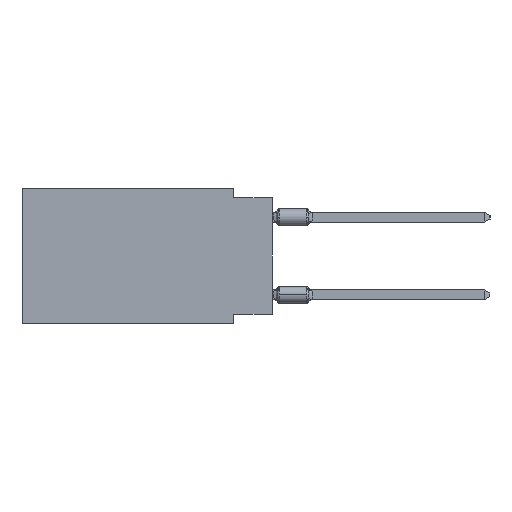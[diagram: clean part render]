
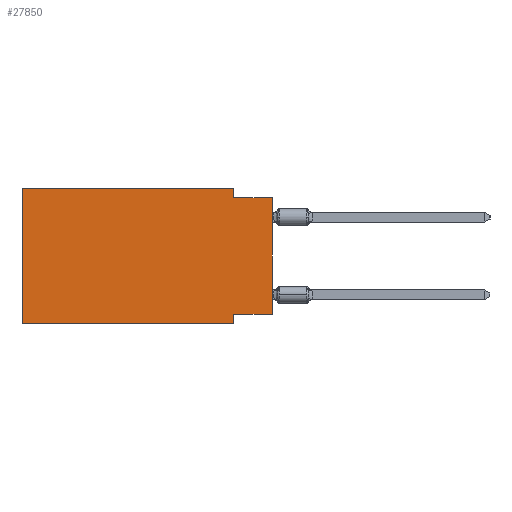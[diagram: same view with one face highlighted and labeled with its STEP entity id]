
A CAD part, left-side view. The second image highlights one B-rep face of the part: STEP entity #27850.
In plain terms, the highlighted planar face has unit normal (-1, 0, 0).
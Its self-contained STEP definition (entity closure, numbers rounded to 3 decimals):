
#627 = CARTESIAN_POINT ( 'NONE',  ( 0., 16.383, 0. ) ) ;
#717 = LINE ( 'NONE', #37979, #37961 ) ;
#2070 = DIRECTION ( 'NONE',  ( 0., 0., -1. ) ) ;
#2710 = CARTESIAN_POINT ( 'NONE',  ( 0., 0., -0.635 ) ) ;
#3313 = EDGE_CURVE ( 'NONE', #24336, #15292, #29046, .T. ) ;
#3346 = LINE ( 'NONE', #28325, #34469 ) ;
#4338 = VECTOR ( 'NONE', #9534, 1000. ) ;
#4487 = CARTESIAN_POINT ( 'NONE',  ( 0., 16.383, -8.89 ) ) ;
#4503 = ORIENTED_EDGE ( 'NONE', *, *, #21146, .F. ) ;
#5913 = EDGE_LOOP ( 'NONE', ( #11246, #27067, #10117, #26167, #31506, #34798, #4503, #7865 ) ) ;
#7865 = ORIENTED_EDGE ( 'NONE', *, *, #16348, .F. ) ;
#8305 = VERTEX_POINT ( 'NONE', #26140 ) ;
#9534 = DIRECTION ( 'NONE',  ( 0., 0., -1. ) ) ;
#9567 = VECTOR ( 'NONE', #10609, 1000. ) ;
#10117 = ORIENTED_EDGE ( 'NONE', *, *, #20426, .F. ) ;
#10234 = DIRECTION ( 'NONE',  ( 0., 0., 1. ) ) ;
#10609 = DIRECTION ( 'NONE',  ( 0., -1., 0. ) ) ;
#10877 = CARTESIAN_POINT ( 'NONE',  ( 0., 16.383, 0. ) ) ;
#11246 = ORIENTED_EDGE ( 'NONE', *, *, #26091, .T. ) ;
#13514 = CARTESIAN_POINT ( 'NONE',  ( 0., 2.54, -0.635 ) ) ;
#14368 = FACE_OUTER_BOUND ( 'NONE', #5913, .T. ) ;
#15292 = VERTEX_POINT ( 'NONE', #19783 ) ;
#15445 = VERTEX_POINT ( 'NONE', #2710 ) ;
#16348 = EDGE_CURVE ( 'NONE', #16973, #19477, #17990, .T. ) ;
#16396 = LINE ( 'NONE', #627, #40320 ) ;
#16973 = VERTEX_POINT ( 'NONE', #21423 ) ;
#17990 = LINE ( 'NONE', #24129, #18792 ) ;
#18792 = VECTOR ( 'NONE', #30476, 1000. ) ;
#19477 = VERTEX_POINT ( 'NONE', #30760 ) ;
#19783 = CARTESIAN_POINT ( 'NONE',  ( 0., 2.54, -8.89 ) ) ;
#20426 = EDGE_CURVE ( 'NONE', #8305, #29395, #22048, .T. ) ;
#20777 = EDGE_CURVE ( 'NONE', #24336, #34880, #16396, .T. ) ;
#21002 = EDGE_CURVE ( 'NONE', #34880, #8305, #40015, .T. ) ;
#21146 = EDGE_CURVE ( 'NONE', #19477, #15292, #3346, .T. ) ;
#21423 = CARTESIAN_POINT ( 'NONE',  ( 0., 0., -8.255 ) ) ;
#22048 = LINE ( 'NONE', #31458, #4338 ) ;
#23381 = DIRECTION ( 'NONE',  ( 1., 0., 0. ) ) ;
#24129 = CARTESIAN_POINT ( 'NONE',  ( 0., 0., -8.255 ) ) ;
#24336 = VERTEX_POINT ( 'NONE', #38128 ) ;
#26091 = EDGE_CURVE ( 'NONE', #16973, #15445, #29679, .T. ) ;
#26140 = CARTESIAN_POINT ( 'NONE',  ( 0., 2.54, 0. ) ) ;
#26167 = ORIENTED_EDGE ( 'NONE', *, *, #21002, .F. ) ;
#26294 = AXIS2_PLACEMENT_3D ( 'NONE', #10877, #23381, #2070 ) ;
#26817 = EDGE_CURVE ( 'NONE', #29395, #15445, #717, .T. ) ;
#27067 = ORIENTED_EDGE ( 'NONE', *, *, #26817, .F. ) ;
#27850 = ADVANCED_FACE ( 'NONE', ( #14368 ), #39336, .F. ) ;
#27952 = CARTESIAN_POINT ( 'NONE',  ( 0., 16.383, 0. ) ) ;
#28325 = CARTESIAN_POINT ( 'NONE',  ( 0., 2.54, -8.89 ) ) ;
#29046 = LINE ( 'NONE', #4487, #9567 ) ;
#29395 = VERTEX_POINT ( 'NONE', #13514 ) ;
#29679 = LINE ( 'NONE', #29889, #33073 ) ;
#29889 = CARTESIAN_POINT ( 'NONE',  ( 0., 0., 0. ) ) ;
#30476 = DIRECTION ( 'NONE',  ( 0., 1., 0. ) ) ;
#30760 = CARTESIAN_POINT ( 'NONE',  ( 0., 2.54, -8.255 ) ) ;
#31409 = DIRECTION ( 'NONE',  ( 0., 0., -1. ) ) ;
#31458 = CARTESIAN_POINT ( 'NONE',  ( 0., 2.54, 0. ) ) ;
#31506 = ORIENTED_EDGE ( 'NONE', *, *, #20777, .F. ) ;
#31670 = CARTESIAN_POINT ( 'NONE',  ( 0., 16.383, 0. ) ) ;
#33012 = DIRECTION ( 'NONE',  ( 0., -1., 0. ) ) ;
#33073 = VECTOR ( 'NONE', #33166, 1000. ) ;
#33166 = DIRECTION ( 'NONE',  ( 0., 0., 1. ) ) ;
#34469 = VECTOR ( 'NONE', #31409, 1000. ) ;
#34798 = ORIENTED_EDGE ( 'NONE', *, *, #3313, .T. ) ;
#34880 = VERTEX_POINT ( 'NONE', #31670 ) ;
#37961 = VECTOR ( 'NONE', #33012, 1000. ) ;
#37979 = CARTESIAN_POINT ( 'NONE',  ( 0., 0., -0.635 ) ) ;
#38128 = CARTESIAN_POINT ( 'NONE',  ( 0., 16.383, -8.89 ) ) ;
#39336 = PLANE ( 'NONE',  #26294 ) ;
#40015 = LINE ( 'NONE', #27952, #40351 ) ;
#40320 = VECTOR ( 'NONE', #10234, 1000. ) ;
#40351 = VECTOR ( 'NONE', #40425, 1000. ) ;
#40425 = DIRECTION ( 'NONE',  ( 0., -1., 0. ) ) ;
